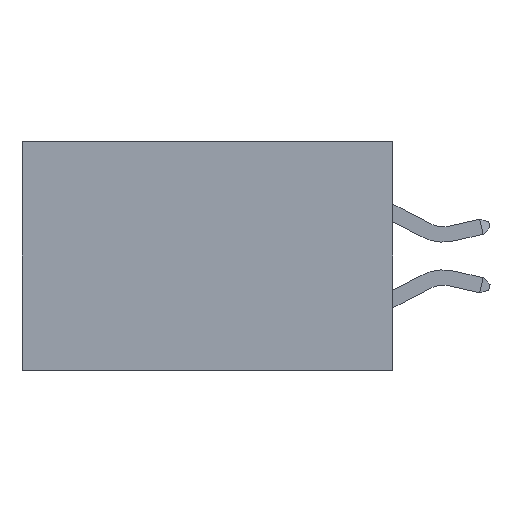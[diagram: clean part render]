
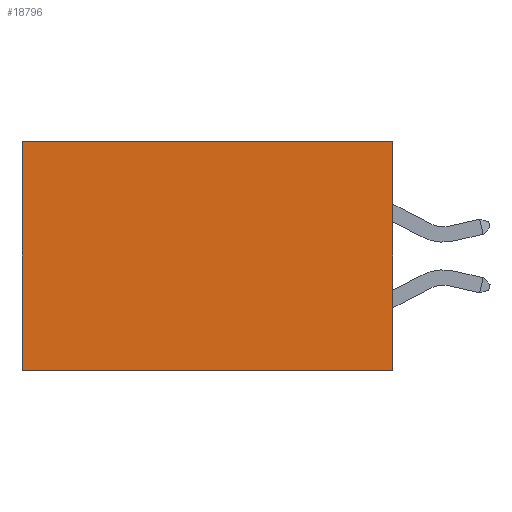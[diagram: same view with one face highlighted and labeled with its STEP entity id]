
A CAD part, left-side view. The second image highlights one B-rep face of the part: STEP entity #18796.
In plain terms, the highlighted planar face has unit normal (-1, 0, 0).
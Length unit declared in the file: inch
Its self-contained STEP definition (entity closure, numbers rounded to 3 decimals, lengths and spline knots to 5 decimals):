
#282 = EDGE_LOOP ( 'NONE', ( #4638, #2548, #18980, #18236 ) ) ;
#740 = EDGE_CURVE ( 'NONE', #11941, #18479, #18362, .T. ) ;
#1463 = CARTESIAN_POINT ( 'NONE',  ( 0.2875, 0.6, 0. ) ) ;
#2548 = ORIENTED_EDGE ( 'NONE', *, *, #5911, .F. ) ;
#3037 = LINE ( 'NONE', #8011, #7650 ) ;
#3257 = CARTESIAN_POINT ( 'NONE',  ( 0.2875, 0.6, -0.37 ) ) ;
#4638 = ORIENTED_EDGE ( 'NONE', *, *, #19070, .T. ) ;
#5911 = EDGE_CURVE ( 'NONE', #18479, #20640, #11266, .T. ) ;
#6319 = DIRECTION ( 'NONE',  ( 0., 0., -1. ) ) ;
#6440 = VERTEX_POINT ( 'NONE', #1463 ) ;
#7650 = VECTOR ( 'NONE', #8101, 39.37008 ) ;
#8011 = CARTESIAN_POINT ( 'NONE',  ( 0.2875, 0.6, 0. ) ) ;
#8083 = DIRECTION ( 'NONE',  ( 0., 1., 0. ) ) ;
#8101 = DIRECTION ( 'NONE',  ( 0., 0., -1. ) ) ;
#8924 = CARTESIAN_POINT ( 'NONE',  ( 0.2875, 0., 0. ) ) ;
#9643 = CARTESIAN_POINT ( 'NONE',  ( 0.2875, 0., -0.37 ) ) ;
#11266 = LINE ( 'NONE', #9643, #14706 ) ;
#11941 = VERTEX_POINT ( 'NONE', #21189 ) ;
#12010 = LINE ( 'NONE', #17846, #21329 ) ;
#12254 = CARTESIAN_POINT ( 'NONE',  ( 0.2875, 0., 0. ) ) ;
#12906 = PLANE ( 'NONE',  #24706 ) ;
#14706 = VECTOR ( 'NONE', #15649, 39.37008 ) ;
#15243 = VECTOR ( 'NONE', #6319, 39.37008 ) ;
#15649 = DIRECTION ( 'NONE',  ( 0., 1., 0. ) ) ;
#16945 = DIRECTION ( 'NONE',  ( 1., 0., 0. ) ) ;
#17659 = FACE_OUTER_BOUND ( 'NONE', #282, .T. ) ;
#17846 = CARTESIAN_POINT ( 'NONE',  ( 0.2875, 0., 0. ) ) ;
#18236 = ORIENTED_EDGE ( 'NONE', *, *, #22767, .T. ) ;
#18255 = CARTESIAN_POINT ( 'NONE',  ( 0.2875, 0., -0.37 ) ) ;
#18362 = LINE ( 'NONE', #12254, #15243 ) ;
#18479 = VERTEX_POINT ( 'NONE', #18255 ) ;
#18796 = ADVANCED_FACE ( 'NONE', ( #17659 ), #12906, .F. ) ;
#18980 = ORIENTED_EDGE ( 'NONE', *, *, #740, .F. ) ;
#19070 = EDGE_CURVE ( 'NONE', #6440, #20640, #3037, .T. ) ;
#20640 = VERTEX_POINT ( 'NONE', #3257 ) ;
#21189 = CARTESIAN_POINT ( 'NONE',  ( 0.2875, 0., 0. ) ) ;
#21329 = VECTOR ( 'NONE', #8083, 39.37008 ) ;
#22767 = EDGE_CURVE ( 'NONE', #11941, #6440, #12010, .T. ) ;
#22860 = DIRECTION ( 'NONE',  ( 0., 0., -1. ) ) ;
#24706 = AXIS2_PLACEMENT_3D ( 'NONE', #8924, #16945, #22860 ) ;
